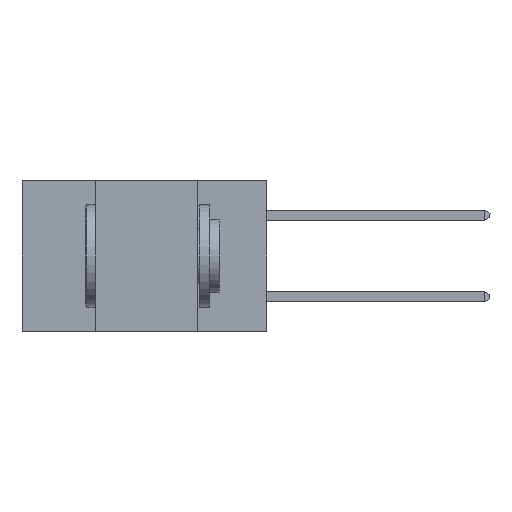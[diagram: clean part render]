
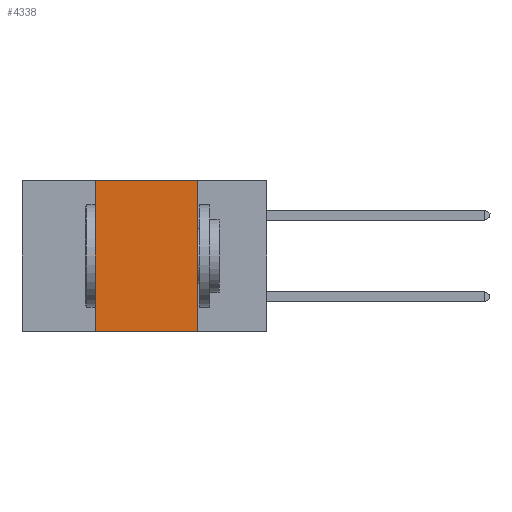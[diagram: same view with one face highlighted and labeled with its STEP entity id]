
A CAD part, left-side view. The second image highlights one B-rep face of the part: STEP entity #4338.
In plain terms, the highlighted planar face has unit normal (-1, 0, 0).
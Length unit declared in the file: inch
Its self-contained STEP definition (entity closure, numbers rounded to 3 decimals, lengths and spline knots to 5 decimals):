
#9 = LINE ( 'NONE', #13692, #3470 ) ;
#187 = DIRECTION ( 'NONE',  ( 0., 0., -1. ) ) ;
#201 = DIRECTION ( 'NONE',  ( 1., 0., 0. ) ) ;
#223 = CARTESIAN_POINT ( 'NONE',  ( 0., 0.6, 0. ) ) ;
#287 = PLANE ( 'NONE',  #3106 ) ;
#342 = CARTESIAN_POINT ( 'NONE',  ( 0., 0.6, -0.37 ) ) ;
#2060 = LINE ( 'NONE', #6938, #14362 ) ;
#2149 = VERTEX_POINT ( 'NONE', #8549 ) ;
#3106 = AXIS2_PLACEMENT_3D ( 'NONE', #223, #201, #187 ) ;
#3470 = VECTOR ( 'NONE', #5606, 39.37008 ) ;
#3594 = EDGE_CURVE ( 'NONE', #10825, #13327, #4302, .T. ) ;
#3596 = CARTESIAN_POINT ( 'NONE',  ( 0., 0.42, -0.37 ) ) ;
#4005 = VERTEX_POINT ( 'NONE', #3596 ) ;
#4302 = LINE ( 'NONE', #8004, #6481 ) ;
#4313 = LINE ( 'NONE', #342, #7602 ) ;
#4338 = ADVANCED_FACE ( 'NONE', ( #13076 ), #287, .F. ) ;
#4365 = ORIENTED_EDGE ( 'NONE', *, *, #9707, .T. ) ;
#4461 = DIRECTION ( 'NONE',  ( 0., 0., 1. ) ) ;
#5606 = DIRECTION ( 'NONE',  ( 0., 0., -1. ) ) ;
#6481 = VECTOR ( 'NONE', #8078, 39.37008 ) ;
#6938 = CARTESIAN_POINT ( 'NONE',  ( 0., 0.42, 0. ) ) ;
#7602 = VECTOR ( 'NONE', #11381, 39.37008 ) ;
#8004 = CARTESIAN_POINT ( 'NONE',  ( 0., 0.6, 0. ) ) ;
#8078 = DIRECTION ( 'NONE',  ( 0., -1., 0. ) ) ;
#8549 = CARTESIAN_POINT ( 'NONE',  ( 0., 0.17, -0.37 ) ) ;
#8917 = ORIENTED_EDGE ( 'NONE', *, *, #3594, .F. ) ;
#9236 = CARTESIAN_POINT ( 'NONE',  ( 0., 0.42, 0. ) ) ;
#9707 = EDGE_CURVE ( 'NONE', #4005, #2149, #4313, .T. ) ;
#10139 = EDGE_LOOP ( 'NONE', ( #14593, #8917, #14959, #4365 ) ) ;
#10825 = VERTEX_POINT ( 'NONE', #9236 ) ;
#11381 = DIRECTION ( 'NONE',  ( 0., -1., 0. ) ) ;
#12452 = CARTESIAN_POINT ( 'NONE',  ( 0., 0.17, 0. ) ) ;
#13076 = FACE_OUTER_BOUND ( 'NONE', #10139, .T. ) ;
#13327 = VERTEX_POINT ( 'NONE', #12452 ) ;
#13692 = CARTESIAN_POINT ( 'NONE',  ( 0., 0.17, 0. ) ) ;
#13974 = EDGE_CURVE ( 'NONE', #4005, #10825, #2060, .T. ) ;
#14362 = VECTOR ( 'NONE', #4461, 39.37008 ) ;
#14549 = EDGE_CURVE ( 'NONE', #13327, #2149, #9, .T. ) ;
#14593 = ORIENTED_EDGE ( 'NONE', *, *, #14549, .F. ) ;
#14959 = ORIENTED_EDGE ( 'NONE', *, *, #13974, .F. ) ;
